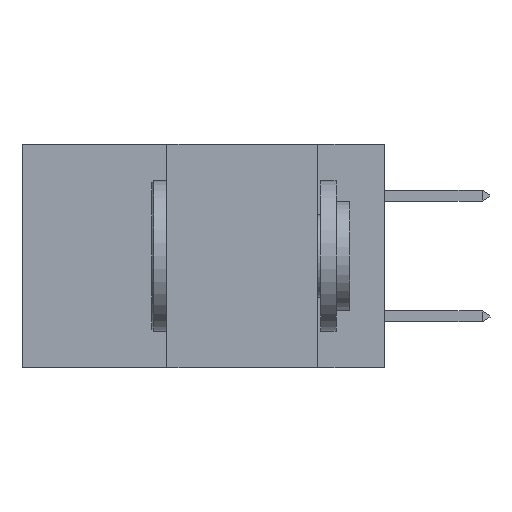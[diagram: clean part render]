
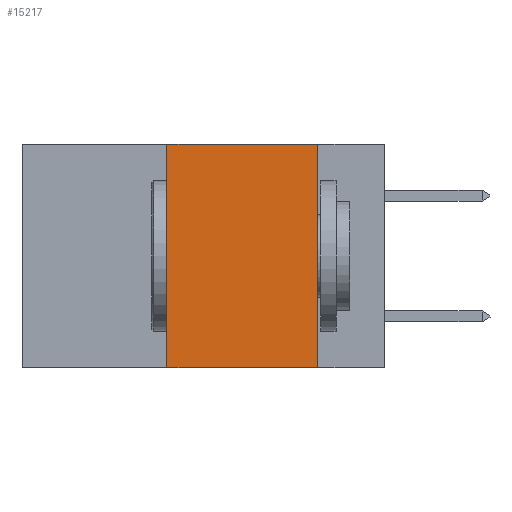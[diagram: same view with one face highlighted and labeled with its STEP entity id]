
A CAD part, left-side view. The second image highlights one B-rep face of the part: STEP entity #15217.
In plain terms, the highlighted planar face has unit normal (-1, 0, 0).
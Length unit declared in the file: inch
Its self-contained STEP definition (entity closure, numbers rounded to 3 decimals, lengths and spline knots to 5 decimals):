
#472 = CARTESIAN_POINT ( 'NONE',  ( 0., 0.11, -0.37 ) ) ;
#698 = VECTOR ( 'NONE', #1390, 39.37008 ) ;
#778 = VERTEX_POINT ( 'NONE', #472 ) ;
#985 = EDGE_CURVE ( 'NONE', #9407, #1494, #14265, .T. ) ;
#1390 = DIRECTION ( 'NONE',  ( 0., -1., 0. ) ) ;
#1494 = VERTEX_POINT ( 'NONE', #3509 ) ;
#1568 = LINE ( 'NONE', #15077, #698 ) ;
#2387 = CARTESIAN_POINT ( 'NONE',  ( 0., 0.11, 0. ) ) ;
#2395 = FACE_OUTER_BOUND ( 'NONE', #4726, .T. ) ;
#2668 = EDGE_CURVE ( 'NONE', #4471, #778, #3776, .T. ) ;
#2743 = VECTOR ( 'NONE', #15532, 39.37008 ) ;
#3065 = ORIENTED_EDGE ( 'NONE', *, *, #10750, .T. ) ;
#3509 = CARTESIAN_POINT ( 'NONE',  ( 0., 0.36, 0. ) ) ;
#3577 = CARTESIAN_POINT ( 'NONE',  ( 0., 0.6, -0.37 ) ) ;
#3776 = LINE ( 'NONE', #2387, #11233 ) ;
#3953 = ORIENTED_EDGE ( 'NONE', *, *, #985, .F. ) ;
#4317 = EDGE_CURVE ( 'NONE', #1494, #4471, #1568, .T. ) ;
#4471 = VERTEX_POINT ( 'NONE', #5260 ) ;
#4726 = EDGE_LOOP ( 'NONE', ( #13051, #7886, #3953, #3065 ) ) ;
#5260 = CARTESIAN_POINT ( 'NONE',  ( 0., 0.11, 0. ) ) ;
#5482 = PLANE ( 'NONE',  #13355 ) ;
#5508 = LINE ( 'NONE', #3577, #2743 ) ;
#6516 = DIRECTION ( 'NONE',  ( 0., 0., -1. ) ) ;
#6913 = CARTESIAN_POINT ( 'NONE',  ( 0., 0.6, 0. ) ) ;
#7886 = ORIENTED_EDGE ( 'NONE', *, *, #4317, .F. ) ;
#8047 = DIRECTION ( 'NONE',  ( 1., 0., 0. ) ) ;
#9407 = VERTEX_POINT ( 'NONE', #15584 ) ;
#10750 = EDGE_CURVE ( 'NONE', #9407, #778, #5508, .T. ) ;
#11091 = CARTESIAN_POINT ( 'NONE',  ( 0., 0.36, 0. ) ) ;
#11233 = VECTOR ( 'NONE', #6516, 39.37008 ) ;
#12454 = DIRECTION ( 'NONE',  ( 0., 0., 1. ) ) ;
#13051 = ORIENTED_EDGE ( 'NONE', *, *, #2668, .F. ) ;
#13355 = AXIS2_PLACEMENT_3D ( 'NONE', #6913, #8047, #14825 ) ;
#14265 = LINE ( 'NONE', #11091, #15324 ) ;
#14825 = DIRECTION ( 'NONE',  ( 0., 0., -1. ) ) ;
#15077 = CARTESIAN_POINT ( 'NONE',  ( 0., 0.6, 0. ) ) ;
#15217 = ADVANCED_FACE ( 'NONE', ( #2395 ), #5482, .F. ) ;
#15324 = VECTOR ( 'NONE', #12454, 39.37008 ) ;
#15532 = DIRECTION ( 'NONE',  ( 0., -1., 0. ) ) ;
#15584 = CARTESIAN_POINT ( 'NONE',  ( 0., 0.36, -0.37 ) ) ;
